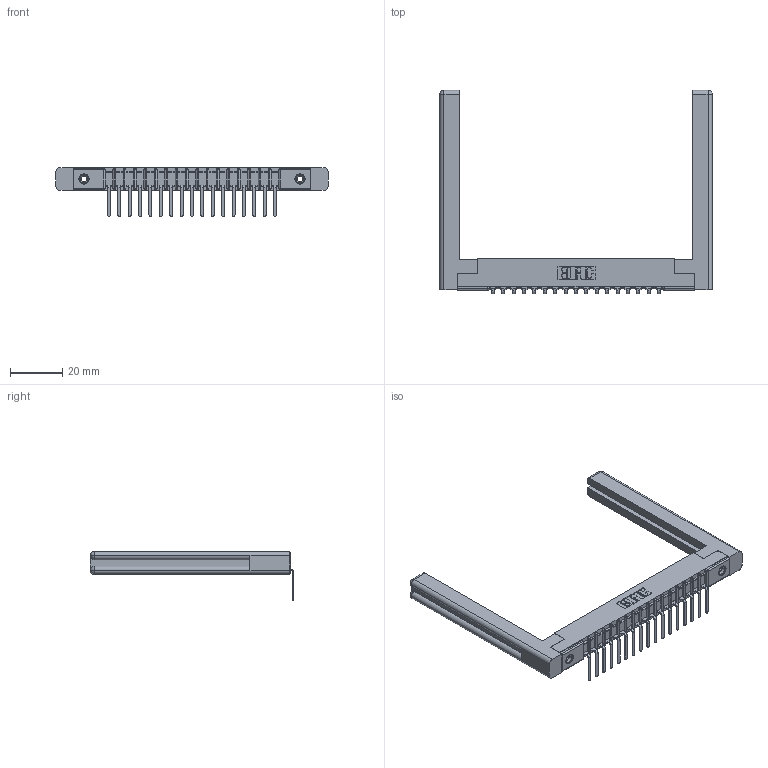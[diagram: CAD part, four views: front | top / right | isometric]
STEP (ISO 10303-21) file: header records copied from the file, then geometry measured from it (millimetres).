
FILE_DESCRIPTION (( 'STEP AP203' ), '1' );
FILE_NAME ('307-017-557-158.STEP', '2019-09-04T22:01:30', ( '' ), ( '' ), 'SwSTEP 2.0', 'SolidWorks 2016', '' );
FILE_SCHEMA (( 'CONFIG_CONTROL_DESIGN' ));
Length unit declared in the file: inch
Products named in the file (5): 307 Part_.156 Dia Mounting Holes; 307-220-058; 307-290-002_557; 345-250-001_345-250-001-102; 307-017-557-158
Assembly tree (22 placements, depth 2):
  307-017-557-158
    307 Part_.156 Dia Mounting Holes
    307-290-002_557  x17
    307-220-058  x2
    345-250-001_345-250-001-102  x2
Bounding box: 103.99 x 77.64 x 18.67 mm (x, y, z)
Volume: 14586.7 mm3; surface area: 17591.7 mm2
Topology: 22 solids, 22 shells, 1604 faces, 4825 edges, 3154 vertices
Faces by surface type: plane 953, cylinder 591, sphere 36, torus 12, cone 12
Entity records: 21143 total; most frequent: CARTESIAN_POINT 3571, ORIENTED_EDGE 3500, DIRECTION 3442, EDGE_CURVE 1750, VECTOR 1324, LINE 1324, VERTEX_POINT 1134, AXIS2_PLACEMENT_3D 1059
